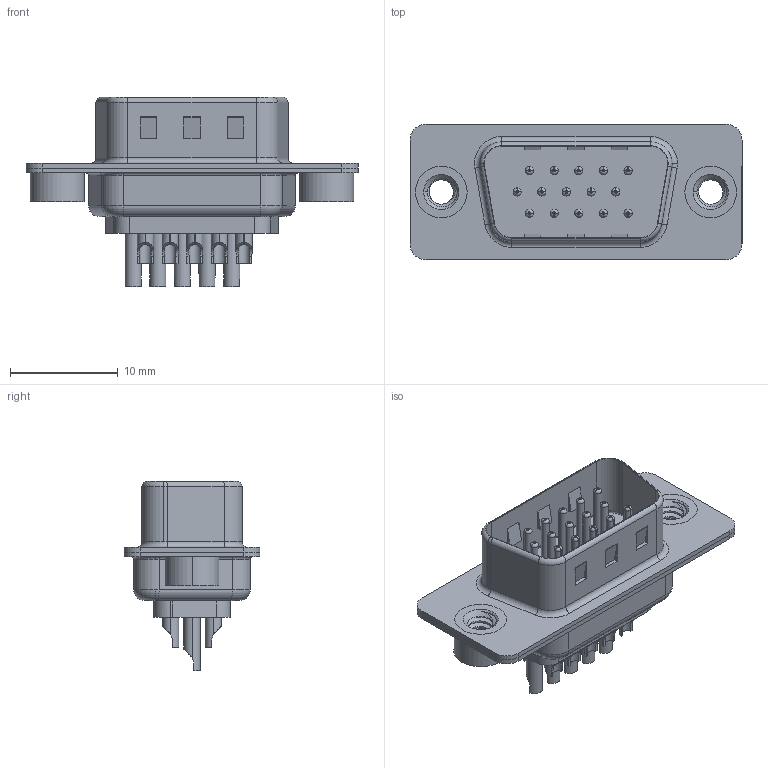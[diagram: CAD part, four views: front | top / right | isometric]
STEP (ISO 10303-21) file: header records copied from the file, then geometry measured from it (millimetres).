
FILE_DESCRIPTION (( 'STEP AP203' ), '1' );
FILE_NAME ('637-015-632-062.STEP', '2020-07-17T23:56:12', ( '' ), ( '' ), 'SwSTEP 2.0', 'SolidWorks 2020', '' );
FILE_SCHEMA (( 'CONFIG_CONTROL_DESIGN' ));
Length unit declared in the file: millimetre
Products named in the file (8): 637 4-40 Threaded Rivet; 637 Contact Row 3_32; 637 Shell Rear_15 Contacts; 637 Shell Front_15 Contacts; 637 Housing_15 Contacts; 637-015-632-062; 637 Contact Row 1_32; 637 Contact Row 2_32
Assembly tree (20 placements, depth 2):
  637-015-632-062
    637 Housing_15 Contacts
    637 Shell Front_15 Contacts
    637 Shell Rear_15 Contacts
    637 Contact Row 1_32  x5
    637 Contact Row 2_32  x5
    637 Contact Row 3_32  x5
    637 4-40 Threaded Rivet  x2
Bounding box: 30.8 x 12.6 x 17.55 mm (x, y, z)
Volume: 1331.8 mm3; surface area: 4778.9 mm2
Topology: 20 solids, 20 shells, 1264 faces, 3217 edges, 2034 vertices
Faces by surface type: cylinder 564, torus 365, plane 317, cone 12, bspline 6
Entity records: 19563 total; most frequent: CARTESIAN_POINT 4508, DIRECTION 3164, ORIENTED_EDGE 2768, EDGE_CURVE 1384, AXIS2_PLACEMENT_3D 1284, VERTEX_POINT 878, CIRCLE 705, EDGE_LOOP 654
